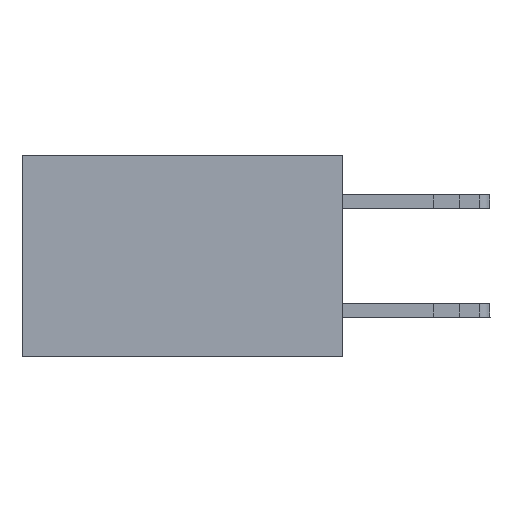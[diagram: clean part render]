
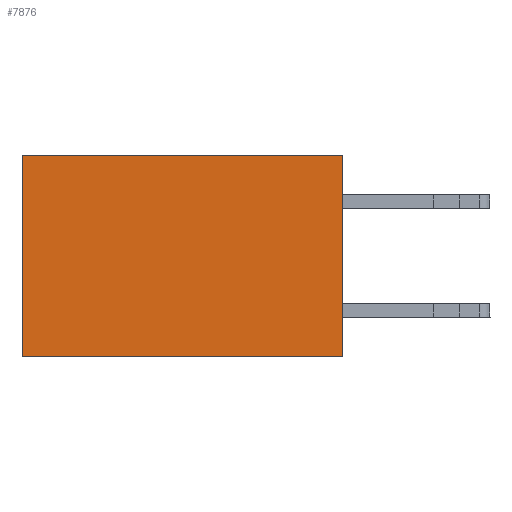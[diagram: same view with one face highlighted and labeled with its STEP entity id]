
A CAD part, left-side view. The second image highlights one B-rep face of the part: STEP entity #7876.
In plain terms, the highlighted planar face has unit normal (-1, 0, 0).
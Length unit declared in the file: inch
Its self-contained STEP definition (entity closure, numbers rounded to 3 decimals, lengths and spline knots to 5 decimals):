
#88 = EDGE_CURVE ( 'NONE', #18958, #12595, #3453, .T. ) ;
#882 = CARTESIAN_POINT ( 'NONE',  ( 0.277, 0.59, -0.37 ) ) ;
#2181 = CARTESIAN_POINT ( 'NONE',  ( 0.277, 0.59, -0.37 ) ) ;
#2736 = CARTESIAN_POINT ( 'NONE',  ( 0.277, 0., -0.37 ) ) ;
#3230 = DIRECTION ( 'NONE',  ( 0., 1., 0. ) ) ;
#3453 = LINE ( 'NONE', #5354, #13014 ) ;
#3579 = VERTEX_POINT ( 'NONE', #6204 ) ;
#4002 = VECTOR ( 'NONE', #16426, 39.37008 ) ;
#4212 = LINE ( 'NONE', #2736, #8943 ) ;
#4743 = VERTEX_POINT ( 'NONE', #882 ) ;
#4794 = EDGE_LOOP ( 'NONE', ( #11161, #21306, #13276, #22331 ) ) ;
#5354 = CARTESIAN_POINT ( 'NONE',  ( 0.277, 0., 0. ) ) ;
#6204 = CARTESIAN_POINT ( 'NONE',  ( 0.277, 0., -0.37 ) ) ;
#6232 = EDGE_CURVE ( 'NONE', #3579, #4743, #4212, .T. ) ;
#7334 = CARTESIAN_POINT ( 'NONE',  ( 0.277, 0., -0.37 ) ) ;
#7876 = ADVANCED_FACE ( 'NONE', ( #21422 ), #14538, .F. ) ;
#8730 = LINE ( 'NONE', #7334, #4002 ) ;
#8839 = CARTESIAN_POINT ( 'NONE',  ( 0.277, 0.59, 0. ) ) ;
#8943 = VECTOR ( 'NONE', #3230, 39.37008 ) ;
#10876 = CARTESIAN_POINT ( 'NONE',  ( 0.277, 0., 0. ) ) ;
#11075 = EDGE_CURVE ( 'NONE', #18958, #3579, #8730, .T. ) ;
#11161 = ORIENTED_EDGE ( 'NONE', *, *, #20543, .T. ) ;
#12595 = VERTEX_POINT ( 'NONE', #8839 ) ;
#12861 = DIRECTION ( 'NONE',  ( 0., 0., -1. ) ) ;
#13014 = VECTOR ( 'NONE', #17191, 39.37008 ) ;
#13151 = LINE ( 'NONE', #2181, #17358 ) ;
#13276 = ORIENTED_EDGE ( 'NONE', *, *, #11075, .F. ) ;
#14413 = DIRECTION ( 'NONE',  ( 0., 0., -1. ) ) ;
#14420 = DIRECTION ( 'NONE',  ( 1., 0., 0. ) ) ;
#14538 = PLANE ( 'NONE',  #19331 ) ;
#14567 = CARTESIAN_POINT ( 'NONE',  ( 0.277, 0., -0.37 ) ) ;
#16426 = DIRECTION ( 'NONE',  ( 0., 0., -1. ) ) ;
#17191 = DIRECTION ( 'NONE',  ( 0., 1., 0. ) ) ;
#17358 = VECTOR ( 'NONE', #12861, 39.37008 ) ;
#18958 = VERTEX_POINT ( 'NONE', #10876 ) ;
#19331 = AXIS2_PLACEMENT_3D ( 'NONE', #14567, #14420, #14413 ) ;
#20543 = EDGE_CURVE ( 'NONE', #12595, #4743, #13151, .T. ) ;
#21306 = ORIENTED_EDGE ( 'NONE', *, *, #6232, .F. ) ;
#21422 = FACE_OUTER_BOUND ( 'NONE', #4794, .T. ) ;
#22331 = ORIENTED_EDGE ( 'NONE', *, *, #88, .T. ) ;
